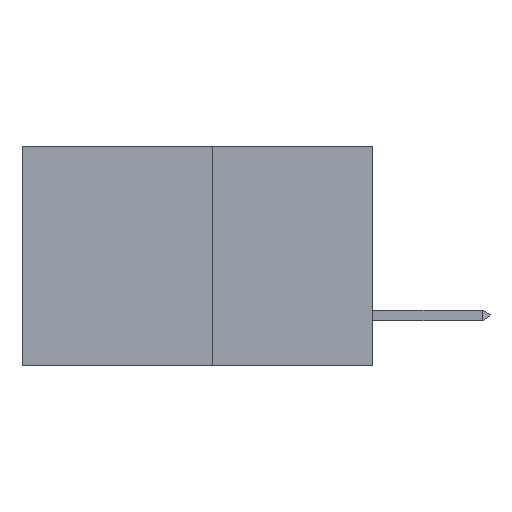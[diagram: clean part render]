
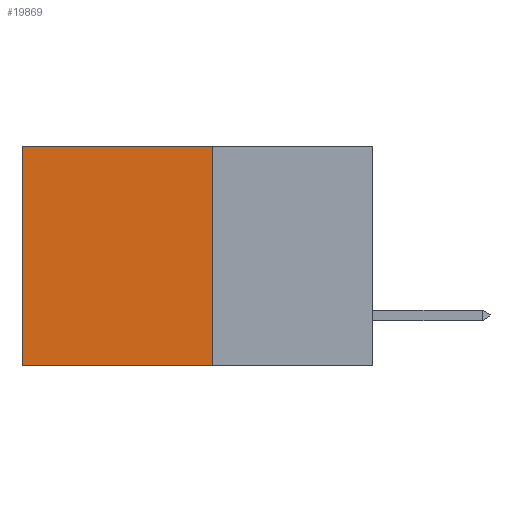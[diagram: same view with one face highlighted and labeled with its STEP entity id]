
A CAD part, left-side view. The second image highlights one B-rep face of the part: STEP entity #19869.
In plain terms, the highlighted planar face has unit normal (-1, 0, 0).
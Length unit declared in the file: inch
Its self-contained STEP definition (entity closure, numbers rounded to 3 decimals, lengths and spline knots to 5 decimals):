
#230 = VECTOR ( 'NONE', #27389, 39.37008 ) ;
#805 = LINE ( 'NONE', #16238, #24255 ) ;
#3533 = EDGE_CURVE ( 'NONE', #15714, #10073, #805, .T. ) ;
#4778 = DIRECTION ( 'NONE',  ( 0., 1., 0. ) ) ;
#5980 = VECTOR ( 'NONE', #14917, 39.37008 ) ;
#6256 = AXIS2_PLACEMENT_3D ( 'NONE', #12304, #27985, #14618 ) ;
#6714 = LINE ( 'NONE', #12596, #5980 ) ;
#7059 = CARTESIAN_POINT ( 'NONE',  ( 0.277, 0.59, -0.37 ) ) ;
#7710 = PLANE ( 'NONE',  #6256 ) ;
#8326 = CARTESIAN_POINT ( 'NONE',  ( 0.277, 0.59, 0. ) ) ;
#10073 = VERTEX_POINT ( 'NONE', #16298 ) ;
#11888 = EDGE_LOOP ( 'NONE', ( #23111, #13860, #14596, #17382 ) ) ;
#12304 = CARTESIAN_POINT ( 'NONE',  ( 0.277, 0.27, -0.37 ) ) ;
#12596 = CARTESIAN_POINT ( 'NONE',  ( 0.277, 0.27, -0.37 ) ) ;
#13286 = FACE_OUTER_BOUND ( 'NONE', #11888, .T. ) ;
#13860 = ORIENTED_EDGE ( 'NONE', *, *, #21816, .F. ) ;
#14596 = ORIENTED_EDGE ( 'NONE', *, *, #3533, .F. ) ;
#14618 = DIRECTION ( 'NONE',  ( 0., 0., -1. ) ) ;
#14917 = DIRECTION ( 'NONE',  ( 0., 1., 0. ) ) ;
#15714 = VERTEX_POINT ( 'NONE', #25925 ) ;
#16238 = CARTESIAN_POINT ( 'NONE',  ( 0.277, 0.27, -0.37 ) ) ;
#16298 = CARTESIAN_POINT ( 'NONE',  ( 0.277, 0.27, -0.37 ) ) ;
#16581 = VERTEX_POINT ( 'NONE', #21841 ) ;
#16905 = EDGE_CURVE ( 'NONE', #24149, #16581, #19872, .T. ) ;
#17382 = ORIENTED_EDGE ( 'NONE', *, *, #21569, .T. ) ;
#17709 = DIRECTION ( 'NONE',  ( 0., 0., -1. ) ) ;
#19205 = VECTOR ( 'NONE', #4778, 39.37008 ) ;
#19869 = ADVANCED_FACE ( 'NONE', ( #13286 ), #7710, .F. ) ;
#19872 = LINE ( 'NONE', #7059, #230 ) ;
#20732 = CARTESIAN_POINT ( 'NONE',  ( 0.277, 0.27, 0. ) ) ;
#21569 = EDGE_CURVE ( 'NONE', #15714, #24149, #25121, .T. ) ;
#21816 = EDGE_CURVE ( 'NONE', #10073, #16581, #6714, .T. ) ;
#21841 = CARTESIAN_POINT ( 'NONE',  ( 0.277, 0.59, -0.37 ) ) ;
#23111 = ORIENTED_EDGE ( 'NONE', *, *, #16905, .T. ) ;
#24149 = VERTEX_POINT ( 'NONE', #8326 ) ;
#24255 = VECTOR ( 'NONE', #17709, 39.37008 ) ;
#25121 = LINE ( 'NONE', #20732, #19205 ) ;
#25925 = CARTESIAN_POINT ( 'NONE',  ( 0.277, 0.27, 0. ) ) ;
#27389 = DIRECTION ( 'NONE',  ( 0., 0., -1. ) ) ;
#27985 = DIRECTION ( 'NONE',  ( 1., 0., 0. ) ) ;
